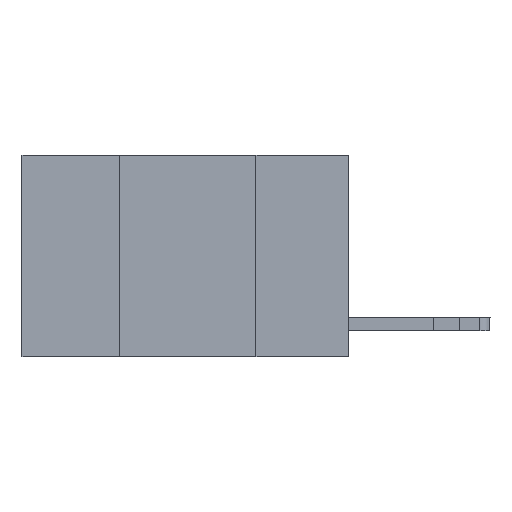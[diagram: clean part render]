
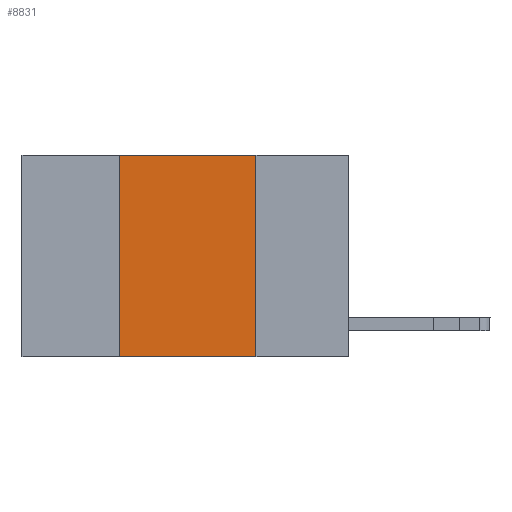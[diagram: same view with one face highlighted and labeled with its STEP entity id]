
A CAD part, left-side view. The second image highlights one B-rep face of the part: STEP entity #8831.
In plain terms, the highlighted planar face has unit normal (-1, 0, 0).
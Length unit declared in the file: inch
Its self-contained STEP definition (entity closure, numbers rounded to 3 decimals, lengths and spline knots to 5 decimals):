
#440 = CARTESIAN_POINT ( 'NONE',  ( 0., 0.17, -0.37 ) ) ;
#487 = CARTESIAN_POINT ( 'NONE',  ( 0., 0.42, 0. ) ) ;
#746 = VERTEX_POINT ( 'NONE', #487 ) ;
#1117 = LINE ( 'NONE', #4209, #5657 ) ;
#1162 = AXIS2_PLACEMENT_3D ( 'NONE', #13306, #11370, #12144 ) ;
#2031 = EDGE_CURVE ( 'NONE', #746, #3119, #1117, .T. ) ;
#2056 = PLANE ( 'NONE',  #1162 ) ;
#2182 = DIRECTION ( 'NONE',  ( 0., -1., 0. ) ) ;
#2186 = VERTEX_POINT ( 'NONE', #440 ) ;
#3119 = VERTEX_POINT ( 'NONE', #13345 ) ;
#3736 = DIRECTION ( 'NONE',  ( 0., 0., -1. ) ) ;
#3822 = FACE_OUTER_BOUND ( 'NONE', #12906, .T. ) ;
#3848 = CARTESIAN_POINT ( 'NONE',  ( 0., 0.6, -0.37 ) ) ;
#4064 = ORIENTED_EDGE ( 'NONE', *, *, #6430, .F. ) ;
#4097 = ORIENTED_EDGE ( 'NONE', *, *, #2031, .F. ) ;
#4209 = CARTESIAN_POINT ( 'NONE',  ( 0., 0.6, 0. ) ) ;
#4220 = VECTOR ( 'NONE', #7981, 39.37008 ) ;
#4434 = VECTOR ( 'NONE', #11357, 39.37008 ) ;
#5182 = VECTOR ( 'NONE', #3736, 39.37008 ) ;
#5657 = VECTOR ( 'NONE', #2182, 39.37008 ) ;
#5902 = LINE ( 'NONE', #6967, #5182 ) ;
#6430 = EDGE_CURVE ( 'NONE', #9862, #746, #13029, .T. ) ;
#6758 = EDGE_CURVE ( 'NONE', #9862, #2186, #13190, .T. ) ;
#6967 = CARTESIAN_POINT ( 'NONE',  ( 0., 0.17, 0. ) ) ;
#7981 = DIRECTION ( 'NONE',  ( 0., -1., 0. ) ) ;
#8215 = CARTESIAN_POINT ( 'NONE',  ( 0., 0.42, 0. ) ) ;
#8787 = ORIENTED_EDGE ( 'NONE', *, *, #6758, .T. ) ;
#8831 = ADVANCED_FACE ( 'NONE', ( #3822 ), #2056, .F. ) ;
#9577 = EDGE_CURVE ( 'NONE', #3119, #2186, #5902, .T. ) ;
#9862 = VERTEX_POINT ( 'NONE', #11869 ) ;
#11121 = ORIENTED_EDGE ( 'NONE', *, *, #9577, .F. ) ;
#11357 = DIRECTION ( 'NONE',  ( 0., 0., 1. ) ) ;
#11370 = DIRECTION ( 'NONE',  ( 1., 0., 0. ) ) ;
#11869 = CARTESIAN_POINT ( 'NONE',  ( 0., 0.42, -0.37 ) ) ;
#12144 = DIRECTION ( 'NONE',  ( 0., 0., -1. ) ) ;
#12906 = EDGE_LOOP ( 'NONE', ( #11121, #4097, #4064, #8787 ) ) ;
#13029 = LINE ( 'NONE', #8215, #4434 ) ;
#13190 = LINE ( 'NONE', #3848, #4220 ) ;
#13306 = CARTESIAN_POINT ( 'NONE',  ( 0., 0.6, 0. ) ) ;
#13345 = CARTESIAN_POINT ( 'NONE',  ( 0., 0.17, 0. ) ) ;
